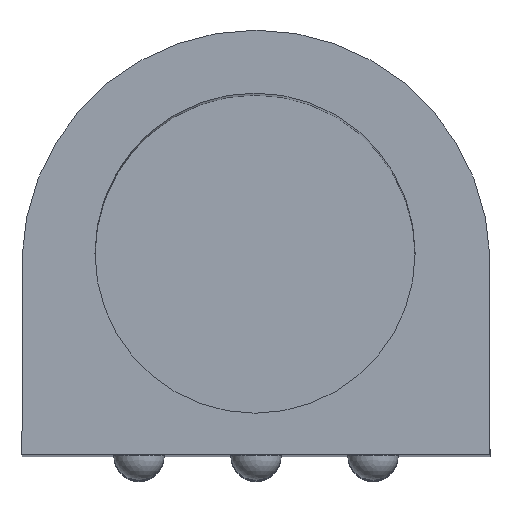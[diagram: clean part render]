
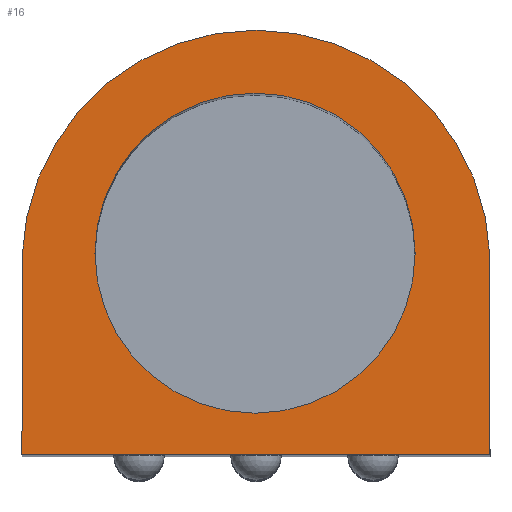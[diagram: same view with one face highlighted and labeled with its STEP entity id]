
A CAD part, top view. The second image highlights one B-rep face of the part: STEP entity #16.
In plain terms, the highlighted planar face has unit normal (0, 0, 1).
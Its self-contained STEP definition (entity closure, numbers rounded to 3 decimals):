
#3 = CARTESIAN_POINT ( 'NONE',  ( -57.618, 39.919, 3.642 ) ) ;
#16 = ADVANCED_FACE ( 'NONE', ( #765, #688 ), #189, .F. ) ;
#17 = CARTESIAN_POINT ( 'NONE',  ( -76.261, 52.942, 3.642 ) ) ;
#18 = VERTEX_POINT ( 'NONE', #374 ) ;
#32 = CARTESIAN_POINT ( 'NONE',  ( -545.084, 24.278, 3.642 ) ) ;
#54 = EDGE_CURVE ( 'NONE', #729, #18, #685, .T. ) ;
#59 = DIRECTION ( 'NONE',  ( 1., 0., 0. ) ) ;
#74 = AXIS2_PLACEMENT_3D ( 'NONE', #529, #526, #522 ) ;
#110 = AXIS2_PLACEMENT_3D ( 'NONE', #668, #666, #660 ) ;
#129 = DIRECTION ( 'NONE',  ( 0., -1., 0. ) ) ;
#189 = PLANE ( 'NONE',  #761 ) ;
#270 = EDGE_LOOP ( 'NONE', ( #988, #712 ) ) ;
#356 = DIRECTION ( 'NONE',  ( 0., 0., 1. ) ) ;
#363 = CIRCLE ( 'NONE', #74, 12.7 ) ;
#367 = VECTOR ( 'NONE', #615, 1000. ) ;
#368 = LINE ( 'NONE', #628, #367 ) ;
#373 = CARTESIAN_POINT ( 'NONE',  ( -94.752, 12.158, 3.642 ) ) ;
#374 = CARTESIAN_POINT ( 'NONE',  ( -94.752, 39.919, 3.642 ) ) ;
#376 = CIRCLE ( 'NONE', #110, 12.7 ) ;
#422 = VECTOR ( 'NONE', #59, 1000. ) ;
#433 = LINE ( 'NONE', #32, #422 ) ;
#441 = VECTOR ( 'NONE', #129, 1000. ) ;
#458 = LINE ( 'NONE', #373, #441 ) ;
#487 = EDGE_CURVE ( 'NONE', #18, #784, #458, .T. ) ;
#520 = DIRECTION ( 'NONE',  ( -1., 0., 0. ) ) ;
#522 = DIRECTION ( 'NONE',  ( -1., 0., 0. ) ) ;
#526 = DIRECTION ( 'NONE',  ( 0., 0., 1. ) ) ;
#529 = CARTESIAN_POINT ( 'NONE',  ( -76.261, 40.242, 3.642 ) ) ;
#544 = CARTESIAN_POINT ( 'NONE',  ( -76.185, 39.361, 3.642 ) ) ;
#615 = DIRECTION ( 'NONE',  ( 0., -1., 0. ) ) ;
#628 = CARTESIAN_POINT ( 'NONE',  ( -57.618, 12.158, 3.642 ) ) ;
#660 = DIRECTION ( 'NONE',  ( -1., 0., 0. ) ) ;
#666 = DIRECTION ( 'NONE',  ( 0., 0., 1. ) ) ;
#668 = CARTESIAN_POINT ( 'NONE',  ( -76.261, 40.242, 3.642 ) ) ;
#674 = DIRECTION ( 'NONE',  ( -1., 0., 0. ) ) ;
#677 = EDGE_LOOP ( 'NONE', ( #973, #837, #909, #863 ) ) ;
#680 = AXIS2_PLACEMENT_3D ( 'NONE', #544, #356, #520 ) ;
#682 = DIRECTION ( 'NONE',  ( 0., 0., -1. ) ) ;
#685 = CIRCLE ( 'NONE', #680, 18.575 ) ;
#688 = FACE_BOUND ( 'NONE', #270, .T. ) ;
#690 = EDGE_CURVE ( 'NONE', #784, #738, #433, .T. ) ;
#698 = VERTEX_POINT ( 'NONE', #17 ) ;
#712 = ORIENTED_EDGE ( 'NONE', *, *, #1003, .F. ) ;
#729 = VERTEX_POINT ( 'NONE', #3 ) ;
#738 = VERTEX_POINT ( 'NONE', #995 ) ;
#761 = AXIS2_PLACEMENT_3D ( 'NONE', #853, #682, #674 ) ;
#765 = FACE_OUTER_BOUND ( 'NONE', #677, .T. ) ;
#784 = VERTEX_POINT ( 'NONE', #972 ) ;
#814 = CARTESIAN_POINT ( 'NONE',  ( -76.261, 27.542, 3.642 ) ) ;
#837 = ORIENTED_EDGE ( 'NONE', *, *, #54, .T. ) ;
#853 = CARTESIAN_POINT ( 'NONE',  ( -395.136, -37.369, 3.642 ) ) ;
#863 = ORIENTED_EDGE ( 'NONE', *, *, #690, .T. ) ;
#876 = VERTEX_POINT ( 'NONE', #814 ) ;
#909 = ORIENTED_EDGE ( 'NONE', *, *, #487, .T. ) ;
#921 = EDGE_CURVE ( 'NONE', #698, #876, #376, .T. ) ;
#969 = EDGE_CURVE ( 'NONE', #729, #738, #368, .T. ) ;
#972 = CARTESIAN_POINT ( 'NONE',  ( -94.752, 24.278, 3.642 ) ) ;
#973 = ORIENTED_EDGE ( 'NONE', *, *, #969, .F. ) ;
#988 = ORIENTED_EDGE ( 'NONE', *, *, #921, .F. ) ;
#995 = CARTESIAN_POINT ( 'NONE',  ( -57.618, 24.278, 3.642 ) ) ;
#1003 = EDGE_CURVE ( 'NONE', #876, #698, #363, .T. ) ;
